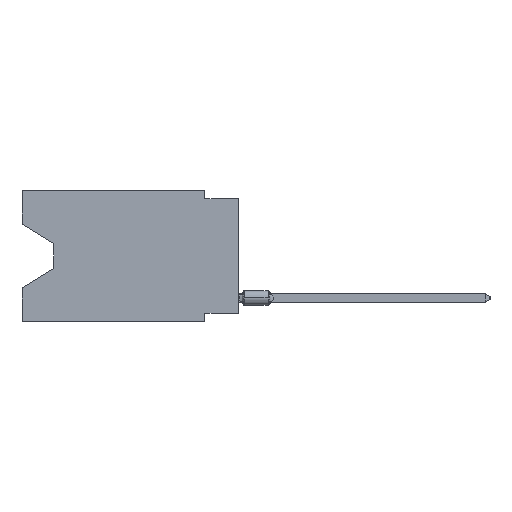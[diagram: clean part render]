
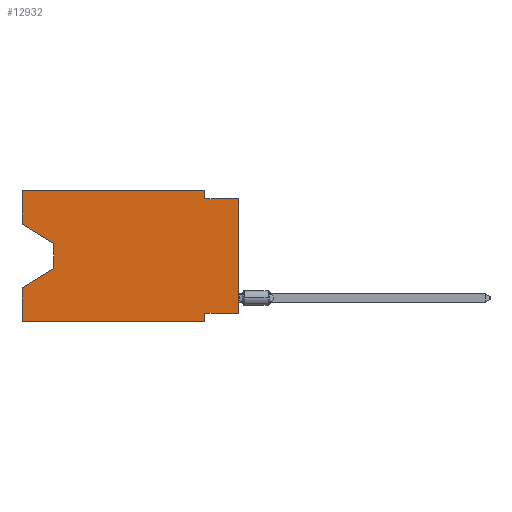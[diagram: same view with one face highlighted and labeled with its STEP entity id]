
A CAD part, left-side view. The second image highlights one B-rep face of the part: STEP entity #12932.
In plain terms, the highlighted planar face has unit normal (-1, 0, 0).
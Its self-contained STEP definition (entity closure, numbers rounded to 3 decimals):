
#448 = CARTESIAN_POINT ( 'NONE',  ( 0., 16.383, -2.546 ) ) ;
#1196 = ORIENTED_EDGE ( 'NONE', *, *, #46497, .T. ) ;
#1370 = ORIENTED_EDGE ( 'NONE', *, *, #37635, .T. ) ;
#3965 = LINE ( 'NONE', #48884, #34109 ) ;
#5996 = CARTESIAN_POINT ( 'NONE',  ( 0., 16.383, 0. ) ) ;
#7423 = ORIENTED_EDGE ( 'NONE', *, *, #23524, .T. ) ;
#7910 = VECTOR ( 'NONE', #55438, 1000. ) ;
#9082 = VECTOR ( 'NONE', #48415, 1000. ) ;
#9242 = LINE ( 'NONE', #42961, #9082 ) ;
#9985 = EDGE_LOOP ( 'NONE', ( #12287, #7423, #1196, #27603, #23091, #53753, #58632, #1370, #15944, #40732, #56860, #49853 ) ) ;
#10813 = CARTESIAN_POINT ( 'NONE',  ( 0., 0., -9.271 ) ) ;
#11012 = VECTOR ( 'NONE', #12375, 1000. ) ;
#11113 = LINE ( 'NONE', #5996, #7910 ) ;
#12287 = ORIENTED_EDGE ( 'NONE', *, *, #60347, .T. ) ;
#12375 = DIRECTION ( 'NONE',  ( 0., 0., -1. ) ) ;
#12932 = ADVANCED_FACE ( 'NONE', ( #32626 ), #47079, .F. ) ;
#14522 = EDGE_CURVE ( 'NONE', #60109, #33281, #11113, .T. ) ;
#14795 = VERTEX_POINT ( 'NONE', #61344 ) ;
#15228 = VECTOR ( 'NONE', #33637, 1000. ) ;
#15944 = ORIENTED_EDGE ( 'NONE', *, *, #37706, .F. ) ;
#16485 = CARTESIAN_POINT ( 'NONE',  ( 0., 2.54, 0. ) ) ;
#17162 = VERTEX_POINT ( 'NONE', #54866 ) ;
#17170 = CARTESIAN_POINT ( 'NONE',  ( 0., 13.97, -4.013 ) ) ;
#17180 = EDGE_CURVE ( 'NONE', #33281, #44142, #50042, .T. ) ;
#18951 = CARTESIAN_POINT ( 'NONE',  ( 0., 13.97, -5.893 ) ) ;
#19561 = CARTESIAN_POINT ( 'NONE',  ( 0., 16.383, 0. ) ) ;
#23091 = ORIENTED_EDGE ( 'NONE', *, *, #36611, .T. ) ;
#23462 = VECTOR ( 'NONE', #50363, 1000. ) ;
#23524 = EDGE_CURVE ( 'NONE', #49732, #46017, #61176, .T. ) ;
#23711 = LINE ( 'NONE', #40373, #36757 ) ;
#24899 = DIRECTION ( 'NONE',  ( 0., 0., -1. ) ) ;
#26123 = LINE ( 'NONE', #16485, #32376 ) ;
#26462 = DIRECTION ( 'NONE',  ( 0., 0., 1. ) ) ;
#26688 = VECTOR ( 'NONE', #52698, 1000. ) ;
#26849 = CARTESIAN_POINT ( 'NONE',  ( 0., 2.54, -0.635 ) ) ;
#27603 = ORIENTED_EDGE ( 'NONE', *, *, #35197, .F. ) ;
#27798 = CARTESIAN_POINT ( 'NONE',  ( 0., 13.97, -5.893 ) ) ;
#29700 = CARTESIAN_POINT ( 'NONE',  ( 0., 16.383, 0. ) ) ;
#30112 = DIRECTION ( 'NONE',  ( 0., -1., 0. ) ) ;
#30158 = CARTESIAN_POINT ( 'NONE',  ( 0., 16.383, -7.36 ) ) ;
#31135 = CARTESIAN_POINT ( 'NONE',  ( 0., 0., -0.635 ) ) ;
#32376 = VECTOR ( 'NONE', #45075, 1000. ) ;
#32626 = FACE_OUTER_BOUND ( 'NONE', #9985, .T. ) ;
#33144 = LINE ( 'NONE', #58495, #38993 ) ;
#33281 = VERTEX_POINT ( 'NONE', #45651 ) ;
#33637 = DIRECTION ( 'NONE',  ( 0., -1., 0. ) ) ;
#34109 = VECTOR ( 'NONE', #43136, 1000. ) ;
#34273 = LINE ( 'NONE', #54170, #15228 ) ;
#35197 = EDGE_CURVE ( 'NONE', #17162, #62211, #50230, .T. ) ;
#36611 = EDGE_CURVE ( 'NONE', #17162, #41894, #34273, .T. ) ;
#36757 = VECTOR ( 'NONE', #30112, 1000. ) ;
#37635 = EDGE_CURVE ( 'NONE', #14795, #49225, #9242, .T. ) ;
#37706 = EDGE_CURVE ( 'NONE', #51161, #49225, #23711, .T. ) ;
#38526 = LINE ( 'NONE', #18951, #26688 ) ;
#38993 = VECTOR ( 'NONE', #52414, 1000. ) ;
#40373 = CARTESIAN_POINT ( 'NONE',  ( 0., 0., -0.635 ) ) ;
#40732 = ORIENTED_EDGE ( 'NONE', *, *, #56576, .F. ) ;
#41894 = VERTEX_POINT ( 'NONE', #46760 ) ;
#42961 = CARTESIAN_POINT ( 'NONE',  ( 0., 0., 0. ) ) ;
#43136 = DIRECTION ( 'NONE',  ( 0., 0., -1. ) ) ;
#43143 = CARTESIAN_POINT ( 'NONE',  ( 0., 13.97, -4.013 ) ) ;
#43839 = DIRECTION ( 'NONE',  ( 1., 0., 0. ) ) ;
#44142 = VERTEX_POINT ( 'NONE', #55968 ) ;
#45075 = DIRECTION ( 'NONE',  ( 0., 0., -1. ) ) ;
#45651 = CARTESIAN_POINT ( 'NONE',  ( 0., 16.383, 0. ) ) ;
#46017 = VERTEX_POINT ( 'NONE', #27798 ) ;
#46497 = EDGE_CURVE ( 'NONE', #46017, #62211, #38526, .T. ) ;
#46760 = CARTESIAN_POINT ( 'NONE',  ( 0., 2.54, -9.906 ) ) ;
#47079 = PLANE ( 'NONE',  #60055 ) ;
#47900 = VECTOR ( 'NONE', #26462, 1000. ) ;
#48415 = DIRECTION ( 'NONE',  ( 0., 0., 1. ) ) ;
#48666 = EDGE_CURVE ( 'NONE', #51977, #41894, #3965, .T. ) ;
#48884 = CARTESIAN_POINT ( 'NONE',  ( 0., 2.54, -9.906 ) ) ;
#49225 = VERTEX_POINT ( 'NONE', #31135 ) ;
#49352 = LINE ( 'NONE', #10813, #55273 ) ;
#49732 = VERTEX_POINT ( 'NONE', #43143 ) ;
#49853 = ORIENTED_EDGE ( 'NONE', *, *, #14522, .F. ) ;
#49990 = DIRECTION ( 'NONE',  ( 0., 1., 0. ) ) ;
#50042 = LINE ( 'NONE', #19561, #23462 ) ;
#50230 = LINE ( 'NONE', #59562, #47900 ) ;
#50363 = DIRECTION ( 'NONE',  ( 0., -1., 0. ) ) ;
#51161 = VERTEX_POINT ( 'NONE', #26849 ) ;
#51977 = VERTEX_POINT ( 'NONE', #54315 ) ;
#52414 = DIRECTION ( 'NONE',  ( 0., -0.855, -0.519 ) ) ;
#52698 = DIRECTION ( 'NONE',  ( 0., 0.855, -0.519 ) ) ;
#53753 = ORIENTED_EDGE ( 'NONE', *, *, #48666, .F. ) ;
#54170 = CARTESIAN_POINT ( 'NONE',  ( 0., 16.383, -9.906 ) ) ;
#54315 = CARTESIAN_POINT ( 'NONE',  ( 0., 2.54, -9.271 ) ) ;
#54866 = CARTESIAN_POINT ( 'NONE',  ( 0., 16.383, -9.906 ) ) ;
#55273 = VECTOR ( 'NONE', #49990, 1000. ) ;
#55438 = DIRECTION ( 'NONE',  ( 0., 0., 1. ) ) ;
#55968 = CARTESIAN_POINT ( 'NONE',  ( 0., 2.54, 0. ) ) ;
#56576 = EDGE_CURVE ( 'NONE', #44142, #51161, #26123, .T. ) ;
#56860 = ORIENTED_EDGE ( 'NONE', *, *, #17180, .F. ) ;
#58495 = CARTESIAN_POINT ( 'NONE',  ( 0., 16.383, -2.546 ) ) ;
#58632 = ORIENTED_EDGE ( 'NONE', *, *, #58994, .F. ) ;
#58994 = EDGE_CURVE ( 'NONE', #14795, #51977, #49352, .T. ) ;
#59562 = CARTESIAN_POINT ( 'NONE',  ( 0., 16.383, 0. ) ) ;
#60055 = AXIS2_PLACEMENT_3D ( 'NONE', #29700, #43839, #24899 ) ;
#60109 = VERTEX_POINT ( 'NONE', #448 ) ;
#60347 = EDGE_CURVE ( 'NONE', #60109, #49732, #33144, .T. ) ;
#61176 = LINE ( 'NONE', #17170, #11012 ) ;
#61344 = CARTESIAN_POINT ( 'NONE',  ( 0., 0., -9.271 ) ) ;
#62211 = VERTEX_POINT ( 'NONE', #30158 ) ;
